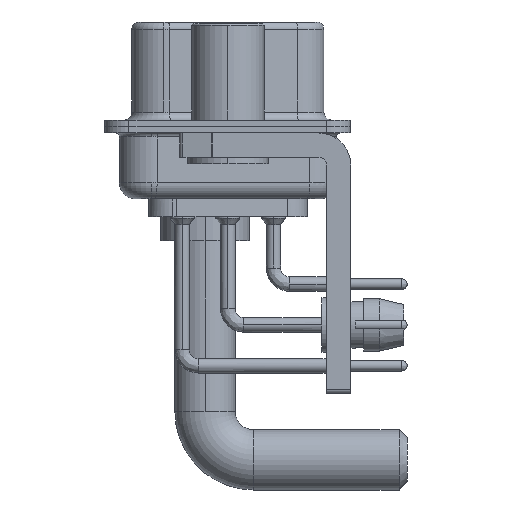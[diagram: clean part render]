
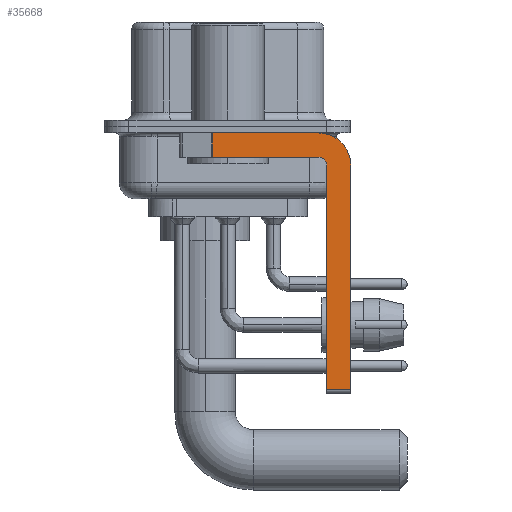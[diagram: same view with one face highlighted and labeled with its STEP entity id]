
A CAD part, left-side view. The second image highlights one B-rep face of the part: STEP entity #35668.
In plain terms, the highlighted planar face has unit normal (-1, 0, 0).
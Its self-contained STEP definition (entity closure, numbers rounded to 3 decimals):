
#105 = VERTEX_POINT ( 'NONE', #17627 ) ;
#108 = CARTESIAN_POINT ( 'NONE',  ( -2.9, -7.65, -2.4 ) ) ;
#1943 = CARTESIAN_POINT ( 'NONE',  ( -2.9, -6.15, -2.4 ) ) ;
#3039 = AXIS2_PLACEMENT_3D ( 'NONE', #13663, #29592, #14457 ) ;
#3765 = DIRECTION ( 'NONE',  ( 0., -1., 0. ) ) ;
#3800 = VERTEX_POINT ( 'NONE', #20614 ) ;
#5883 = DIRECTION ( 'NONE',  ( 0., 1., 0. ) ) ;
#6222 = DIRECTION ( 'NONE',  ( 0., 0., -1. ) ) ;
#6488 = VERTEX_POINT ( 'NONE', #20557 ) ;
#7485 = ORIENTED_EDGE ( 'NONE', *, *, #22036, .F. ) ;
#7653 = VECTOR ( 'NONE', #3765, 1000. ) ;
#8219 = CARTESIAN_POINT ( 'NONE',  ( -2.9, 0.978, -1.9 ) ) ;
#8299 = VECTOR ( 'NONE', #20701, 1000. ) ;
#8849 = CARTESIAN_POINT ( 'NONE',  ( -2.9, -5.65, -2.4 ) ) ;
#9341 = VECTOR ( 'NONE', #11797, 1000. ) ;
#9773 = EDGE_CURVE ( 'NONE', #15440, #6488, #14636, .T. ) ;
#10343 = ORIENTED_EDGE ( 'NONE', *, *, #23845, .F. ) ;
#10615 = ORIENTED_EDGE ( 'NONE', *, *, #9773, .T. ) ;
#11096 = ORIENTED_EDGE ( 'NONE', *, *, #38949, .F. ) ;
#11797 = DIRECTION ( 'NONE',  ( 0., -1., 0. ) ) ;
#12406 = LINE ( 'NONE', #36929, #23403 ) ;
#13658 = AXIS2_PLACEMENT_3D ( 'NONE', #8849, #21313, #35397 ) ;
#13663 = CARTESIAN_POINT ( 'NONE',  ( -2.9, -5.65, -2.4 ) ) ;
#14096 = CIRCLE ( 'NONE', #3039, 0.5 ) ;
#14429 = CARTESIAN_POINT ( 'NONE',  ( -2.9, -5.65, -16.35 ) ) ;
#14457 = DIRECTION ( 'NONE',  ( 0., 0., 1. ) ) ;
#14636 = LINE ( 'NONE', #14429, #9341 ) ;
#14693 = EDGE_CURVE ( 'NONE', #105, #20523, #22556, .T. ) ;
#14763 = LINE ( 'NONE', #39698, #8299 ) ;
#14778 = CARTESIAN_POINT ( 'NONE',  ( -2.9, -5.65, -0.4 ) ) ;
#14887 = VECTOR ( 'NONE', #29359, 1000. ) ;
#15260 = VERTEX_POINT ( 'NONE', #14778 ) ;
#15440 = VERTEX_POINT ( 'NONE', #37057 ) ;
#16024 = CARTESIAN_POINT ( 'NONE',  ( -2.9, 3., -0.4 ) ) ;
#16225 = CIRCLE ( 'NONE', #16900, 2. ) ;
#16900 = AXIS2_PLACEMENT_3D ( 'NONE', #37500, #37700, #25021 ) ;
#17291 = LINE ( 'NONE', #20559, #14887 ) ;
#17627 = CARTESIAN_POINT ( 'NONE',  ( -2.9, 0.978, -0.4 ) ) ;
#18914 = VERTEX_POINT ( 'NONE', #1943 ) ;
#20408 = EDGE_CURVE ( 'NONE', #105, #15260, #35431, .T. ) ;
#20523 = VERTEX_POINT ( 'NONE', #8219 ) ;
#20557 = CARTESIAN_POINT ( 'NONE',  ( -2.9, -7.65, -16.35 ) ) ;
#20559 = CARTESIAN_POINT ( 'NONE',  ( -2.9, -6.15, -16.6 ) ) ;
#20614 = CARTESIAN_POINT ( 'NONE',  ( -2.9, -5.65, -1.9 ) ) ;
#20701 = DIRECTION ( 'NONE',  ( 0., 0., -1. ) ) ;
#21313 = DIRECTION ( 'NONE',  ( 1., 0., 0. ) ) ;
#22036 = EDGE_CURVE ( 'NONE', #3800, #20523, #12406, .T. ) ;
#22556 = LINE ( 'NONE', #35014, #26273 ) ;
#23394 = ORIENTED_EDGE ( 'NONE', *, *, #14693, .T. ) ;
#23403 = VECTOR ( 'NONE', #5883, 1000. ) ;
#23808 = VERTEX_POINT ( 'NONE', #108 ) ;
#23845 = EDGE_CURVE ( 'NONE', #15260, #23808, #16225, .T. ) ;
#24739 = ORIENTED_EDGE ( 'NONE', *, *, #20408, .F. ) ;
#25021 = DIRECTION ( 'NONE',  ( 0., 0., -1. ) ) ;
#26273 = VECTOR ( 'NONE', #6222, 1000. ) ;
#27541 = ORIENTED_EDGE ( 'NONE', *, *, #29198, .F. ) ;
#29198 = EDGE_CURVE ( 'NONE', #18914, #3800, #14096, .T. ) ;
#29359 = DIRECTION ( 'NONE',  ( 0., 0., 1. ) ) ;
#29592 = DIRECTION ( 'NONE',  ( -1., 0., 0. ) ) ;
#29972 = EDGE_LOOP ( 'NONE', ( #24739, #23394, #7485, #27541, #11096, #10615, #34899, #10343 ) ) ;
#34899 = ORIENTED_EDGE ( 'NONE', *, *, #38232, .F. ) ;
#35014 = CARTESIAN_POINT ( 'NONE',  ( -2.9, 0.978, -1.9 ) ) ;
#35397 = DIRECTION ( 'NONE',  ( 0., 0., -1. ) ) ;
#35431 = LINE ( 'NONE', #16024, #7653 ) ;
#35668 = ADVANCED_FACE ( 'NONE', ( #39910 ), #36838, .F. ) ;
#36838 = PLANE ( 'NONE',  #13658 ) ;
#36929 = CARTESIAN_POINT ( 'NONE',  ( -2.9, -5.65, -1.9 ) ) ;
#37057 = CARTESIAN_POINT ( 'NONE',  ( -2.9, -6.15, -16.35 ) ) ;
#37500 = CARTESIAN_POINT ( 'NONE',  ( -2.9, -5.65, -2.4 ) ) ;
#37700 = DIRECTION ( 'NONE',  ( 1., 0., 0. ) ) ;
#38232 = EDGE_CURVE ( 'NONE', #23808, #6488, #14763, .T. ) ;
#38949 = EDGE_CURVE ( 'NONE', #15440, #18914, #17291, .T. ) ;
#39698 = CARTESIAN_POINT ( 'NONE',  ( -2.9, -7.65, -2.4 ) ) ;
#39910 = FACE_OUTER_BOUND ( 'NONE', #29972, .T. ) ;
